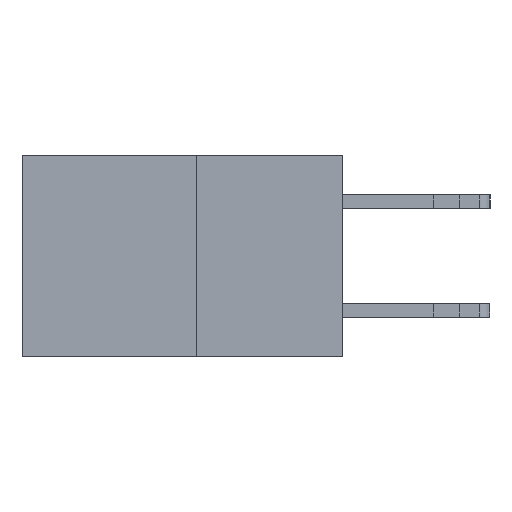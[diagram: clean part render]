
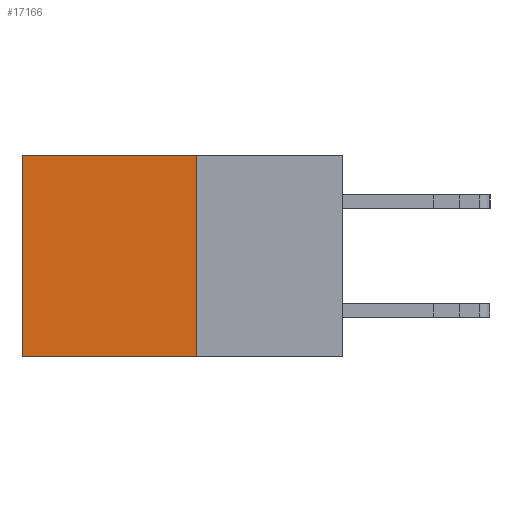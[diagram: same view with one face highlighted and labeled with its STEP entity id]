
A CAD part, left-side view. The second image highlights one B-rep face of the part: STEP entity #17166.
In plain terms, the highlighted planar face has unit normal (-1, 0, 0).
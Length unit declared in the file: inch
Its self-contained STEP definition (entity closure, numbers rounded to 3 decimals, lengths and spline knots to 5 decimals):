
#682 = CARTESIAN_POINT ( 'NONE',  ( 0.277, 0.27, -0.37 ) ) ;
#1294 = LINE ( 'NONE', #8469, #18854 ) ;
#1401 = ORIENTED_EDGE ( 'NONE', *, *, #6733, .T. ) ;
#1744 = CARTESIAN_POINT ( 'NONE',  ( 0.277, 0.27, -0.37 ) ) ;
#1779 = DIRECTION ( 'NONE',  ( 0., 1., 0. ) ) ;
#3452 = DIRECTION ( 'NONE',  ( 1., 0., 0. ) ) ;
#4630 = LINE ( 'NONE', #21390, #17681 ) ;
#4958 = VERTEX_POINT ( 'NONE', #11550 ) ;
#5603 = VECTOR ( 'NONE', #7576, 39.37008 ) ;
#5859 = CARTESIAN_POINT ( 'NONE',  ( 0.277, 0.27, 0. ) ) ;
#6663 = VECTOR ( 'NONE', #7982, 39.37008 ) ;
#6733 = EDGE_CURVE ( 'NONE', #18776, #14488, #20792, .T. ) ;
#6822 = CARTESIAN_POINT ( 'NONE',  ( 0.277, 0.59, 0. ) ) ;
#7576 = DIRECTION ( 'NONE',  ( 0., 1., 0. ) ) ;
#7982 = DIRECTION ( 'NONE',  ( 0., 0., -1. ) ) ;
#8167 = ORIENTED_EDGE ( 'NONE', *, *, #16899, .F. ) ;
#8179 = CARTESIAN_POINT ( 'NONE',  ( 0.277, 0.59, -0.37 ) ) ;
#8469 = CARTESIAN_POINT ( 'NONE',  ( 0.277, 0.27, -0.37 ) ) ;
#11068 = AXIS2_PLACEMENT_3D ( 'NONE', #1744, #3452, #15333 ) ;
#11550 = CARTESIAN_POINT ( 'NONE',  ( 0.277, 0.27, 0. ) ) ;
#11863 = EDGE_CURVE ( 'NONE', #16132, #14488, #1294, .T. ) ;
#12922 = DIRECTION ( 'NONE',  ( 0., 0., -1. ) ) ;
#14488 = VERTEX_POINT ( 'NONE', #15287 ) ;
#14764 = EDGE_CURVE ( 'NONE', #4958, #18776, #19729, .T. ) ;
#15261 = PLANE ( 'NONE',  #11068 ) ;
#15287 = CARTESIAN_POINT ( 'NONE',  ( 0.277, 0.59, -0.37 ) ) ;
#15333 = DIRECTION ( 'NONE',  ( 0., 0., -1. ) ) ;
#16132 = VERTEX_POINT ( 'NONE', #682 ) ;
#16337 = ORIENTED_EDGE ( 'NONE', *, *, #14764, .T. ) ;
#16899 = EDGE_CURVE ( 'NONE', #4958, #16132, #4630, .T. ) ;
#17166 = ADVANCED_FACE ( 'NONE', ( #20824 ), #15261, .F. ) ;
#17681 = VECTOR ( 'NONE', #12922, 39.37008 ) ;
#18776 = VERTEX_POINT ( 'NONE', #6822 ) ;
#18854 = VECTOR ( 'NONE', #1779, 39.37008 ) ;
#19729 = LINE ( 'NONE', #5859, #5603 ) ;
#20578 = ORIENTED_EDGE ( 'NONE', *, *, #11863, .F. ) ;
#20792 = LINE ( 'NONE', #8179, #6663 ) ;
#20824 = FACE_OUTER_BOUND ( 'NONE', #21117, .T. ) ;
#21117 = EDGE_LOOP ( 'NONE', ( #1401, #20578, #8167, #16337 ) ) ;
#21390 = CARTESIAN_POINT ( 'NONE',  ( 0.277, 0.27, -0.37 ) ) ;
